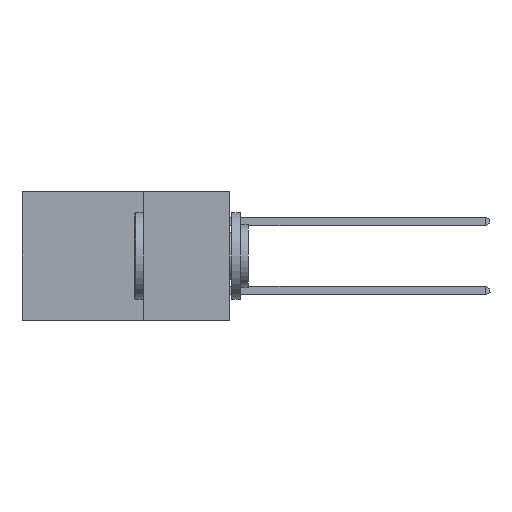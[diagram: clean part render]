
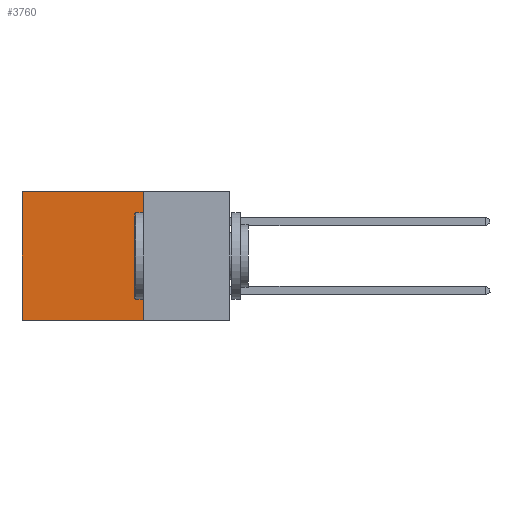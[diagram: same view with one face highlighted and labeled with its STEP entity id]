
A CAD part, left-side view. The second image highlights one B-rep face of the part: STEP entity #3760.
In plain terms, the highlighted planar face has unit normal (-1, 0, 0).
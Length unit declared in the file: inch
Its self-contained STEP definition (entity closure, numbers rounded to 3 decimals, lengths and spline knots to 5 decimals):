
#742 = EDGE_LOOP ( 'NONE', ( #4708, #15551, #3972, #20046 ) ) ;
#1418 = DIRECTION ( 'NONE',  ( 0., 1., 0. ) ) ;
#1879 = EDGE_CURVE ( 'NONE', #19904, #23863, #21742, .T. ) ;
#2640 = DIRECTION ( 'NONE',  ( 1., 0., 0. ) ) ;
#3760 = ADVANCED_FACE ( 'NONE', ( #20506 ), #17481, .F. ) ;
#3972 = ORIENTED_EDGE ( 'NONE', *, *, #1879, .F. ) ;
#4280 = AXIS2_PLACEMENT_3D ( 'NONE', #8084, #2640, #4293 ) ;
#4293 = DIRECTION ( 'NONE',  ( 0., 0., -1. ) ) ;
#4708 = ORIENTED_EDGE ( 'NONE', *, *, #7782, .T. ) ;
#5474 = CARTESIAN_POINT ( 'NONE',  ( 0.298, 0.6, 0. ) ) ;
#5554 = CARTESIAN_POINT ( 'NONE',  ( 0.298, 0.25, 0. ) ) ;
#7365 = VECTOR ( 'NONE', #10730, 39.37008 ) ;
#7554 = VECTOR ( 'NONE', #19679, 39.37008 ) ;
#7782 = EDGE_CURVE ( 'NONE', #17058, #16840, #23655, .T. ) ;
#8084 = CARTESIAN_POINT ( 'NONE',  ( 0.298, 0.25, 0. ) ) ;
#8953 = CARTESIAN_POINT ( 'NONE',  ( 0.298, 0.6, 0. ) ) ;
#9858 = CARTESIAN_POINT ( 'NONE',  ( 0.298, 0.6, -0.37 ) ) ;
#9874 = LINE ( 'NONE', #17974, #10766 ) ;
#10730 = DIRECTION ( 'NONE',  ( 0., 1., 0. ) ) ;
#10754 = EDGE_CURVE ( 'NONE', #19904, #17058, #9874, .T. ) ;
#10766 = VECTOR ( 'NONE', #1418, 39.37008 ) ;
#14289 = CARTESIAN_POINT ( 'NONE',  ( 0.298, 0.25, -0.37 ) ) ;
#14769 = DIRECTION ( 'NONE',  ( 0., 0., -1. ) ) ;
#15551 = ORIENTED_EDGE ( 'NONE', *, *, #18607, .F. ) ;
#15855 = CARTESIAN_POINT ( 'NONE',  ( 0.298, 0.25, 0. ) ) ;
#16840 = VERTEX_POINT ( 'NONE', #9858 ) ;
#16935 = LINE ( 'NONE', #14289, #7365 ) ;
#17058 = VERTEX_POINT ( 'NONE', #5474 ) ;
#17481 = PLANE ( 'NONE',  #4280 ) ;
#17974 = CARTESIAN_POINT ( 'NONE',  ( 0.298, 0.25, 0. ) ) ;
#18097 = CARTESIAN_POINT ( 'NONE',  ( 0.298, 0.25, -0.37 ) ) ;
#18607 = EDGE_CURVE ( 'NONE', #23863, #16840, #16935, .T. ) ;
#18746 = VECTOR ( 'NONE', #14769, 39.37008 ) ;
#19679 = DIRECTION ( 'NONE',  ( 0., 0., -1. ) ) ;
#19904 = VERTEX_POINT ( 'NONE', #5554 ) ;
#20046 = ORIENTED_EDGE ( 'NONE', *, *, #10754, .T. ) ;
#20506 = FACE_OUTER_BOUND ( 'NONE', #742, .T. ) ;
#21742 = LINE ( 'NONE', #15855, #7554 ) ;
#23655 = LINE ( 'NONE', #8953, #18746 ) ;
#23863 = VERTEX_POINT ( 'NONE', #18097 ) ;
